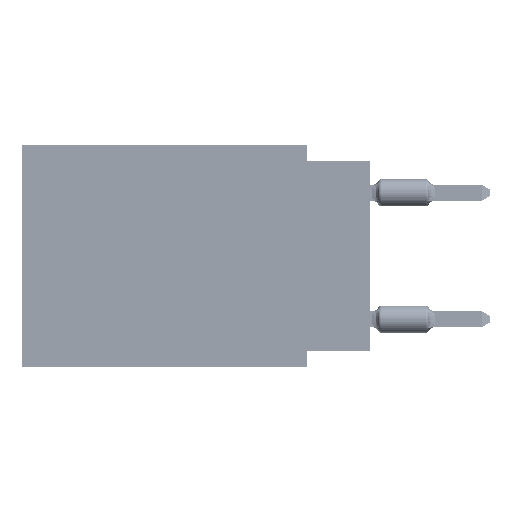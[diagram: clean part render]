
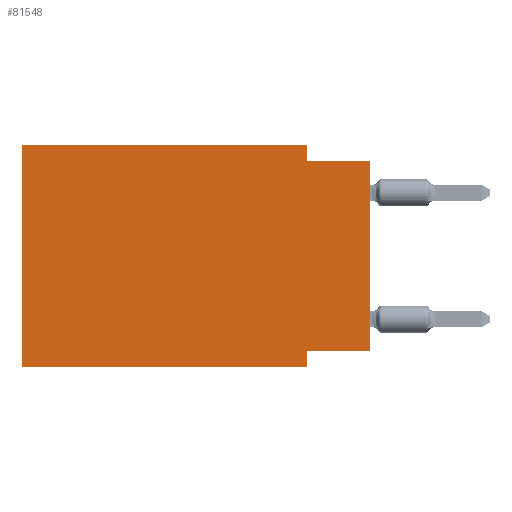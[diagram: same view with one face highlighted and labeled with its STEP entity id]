
A CAD part, left-side view. The second image highlights one B-rep face of the part: STEP entity #81548.
In plain terms, the highlighted planar face has unit normal (-1, 0, 0).
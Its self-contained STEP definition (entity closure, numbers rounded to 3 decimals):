
#2024 = ORIENTED_EDGE ( 'NONE', *, *, #3509, .F. ) ;
#3143 = AXIS2_PLACEMENT_3D ( 'NONE', #29264, #36992, #66428 ) ;
#3509 = EDGE_CURVE ( 'NONE', #34362, #30360, #39210, .T. ) ;
#3958 = EDGE_CURVE ( 'NONE', #67403, #28481, #68541, .T. ) ;
#7052 = FACE_OUTER_BOUND ( 'NONE', #92737, .T. ) ;
#7469 = CARTESIAN_POINT ( 'NONE',  ( 0., 2.54, 0. ) ) ;
#8849 = VERTEX_POINT ( 'NONE', #11582 ) ;
#9757 = LINE ( 'NONE', #38260, #19211 ) ;
#11582 = CARTESIAN_POINT ( 'NONE',  ( 0., 2.54, -8.255 ) ) ;
#16676 = DIRECTION ( 'NONE',  ( 0., -1., 0. ) ) ;
#19211 = VECTOR ( 'NONE', #69609, 1000. ) ;
#26315 = CARTESIAN_POINT ( 'NONE',  ( 0., 13.97, -8.89 ) ) ;
#27398 = EDGE_CURVE ( 'NONE', #8849, #62726, #47108, .T. ) ;
#28058 = ORIENTED_EDGE ( 'NONE', *, *, #45153, .T. ) ;
#28481 = VERTEX_POINT ( 'NONE', #76829 ) ;
#29264 = CARTESIAN_POINT ( 'NONE',  ( 0., 13.97, 0. ) ) ;
#30360 = VERTEX_POINT ( 'NONE', #59349 ) ;
#31973 = CARTESIAN_POINT ( 'NONE',  ( 0., 13.97, 0. ) ) ;
#32003 = CARTESIAN_POINT ( 'NONE',  ( 0., 2.54, 0. ) ) ;
#33080 = VERTEX_POINT ( 'NONE', #58321 ) ;
#34362 = VERTEX_POINT ( 'NONE', #39349 ) ;
#35108 = ORIENTED_EDGE ( 'NONE', *, *, #39375, .F. ) ;
#35407 = VECTOR ( 'NONE', #42680, 1000. ) ;
#36440 = VECTOR ( 'NONE', #90115, 1000. ) ;
#36992 = DIRECTION ( 'NONE',  ( 1., 0., 0. ) ) ;
#38260 = CARTESIAN_POINT ( 'NONE',  ( 0., 13.97, 0. ) ) ;
#38463 = CARTESIAN_POINT ( 'NONE',  ( 0., 2.54, -8.89 ) ) ;
#39210 = LINE ( 'NONE', #31973, #61762 ) ;
#39349 = CARTESIAN_POINT ( 'NONE',  ( 0., 13.97, -8.89 ) ) ;
#39375 = EDGE_CURVE ( 'NONE', #30360, #82063, #9757, .T. ) ;
#40189 = ORIENTED_EDGE ( 'NONE', *, *, #27398, .F. ) ;
#42680 = DIRECTION ( 'NONE',  ( 0., 1., 0. ) ) ;
#43485 = ORIENTED_EDGE ( 'NONE', *, *, #44630, .T. ) ;
#44630 = EDGE_CURVE ( 'NONE', #34362, #62726, #63002, .T. ) ;
#45153 = EDGE_CURVE ( 'NONE', #33080, #28481, #72029, .T. ) ;
#46510 = LINE ( 'NONE', #7469, #48890 ) ;
#47108 = LINE ( 'NONE', #38463, #36440 ) ;
#48890 = VECTOR ( 'NONE', #70161, 1000. ) ;
#56105 = ORIENTED_EDGE ( 'NONE', *, *, #71677, .F. ) ;
#56377 = VECTOR ( 'NONE', #85104, 1000. ) ;
#57176 = CARTESIAN_POINT ( 'NONE',  ( 0., 0., -8.255 ) ) ;
#58133 = CARTESIAN_POINT ( 'NONE',  ( 0., 2.54, -0.635 ) ) ;
#58214 = PLANE ( 'NONE',  #3143 ) ;
#58321 = CARTESIAN_POINT ( 'NONE',  ( 0., 0., -8.255 ) ) ;
#59349 = CARTESIAN_POINT ( 'NONE',  ( 0., 13.97, 0. ) ) ;
#59772 = ORIENTED_EDGE ( 'NONE', *, *, #76416, .F. ) ;
#61291 = CARTESIAN_POINT ( 'NONE',  ( 0., 0., -0.635 ) ) ;
#61762 = VECTOR ( 'NONE', #68650, 1000. ) ;
#62726 = VERTEX_POINT ( 'NONE', #63433 ) ;
#63002 = LINE ( 'NONE', #26315, #79534 ) ;
#63433 = CARTESIAN_POINT ( 'NONE',  ( 0., 2.54, -8.89 ) ) ;
#66320 = LINE ( 'NONE', #57176, #35407 ) ;
#66428 = DIRECTION ( 'NONE',  ( 0., 0., -1. ) ) ;
#67403 = VERTEX_POINT ( 'NONE', #58133 ) ;
#68541 = LINE ( 'NONE', #61291, #74178 ) ;
#68650 = DIRECTION ( 'NONE',  ( 0., 0., 1. ) ) ;
#69609 = DIRECTION ( 'NONE',  ( 0., -1., 0. ) ) ;
#70161 = DIRECTION ( 'NONE',  ( 0., 0., -1. ) ) ;
#71677 = EDGE_CURVE ( 'NONE', #33080, #8849, #66320, .T. ) ;
#72029 = LINE ( 'NONE', #94241, #56377 ) ;
#74178 = VECTOR ( 'NONE', #90757, 1000. ) ;
#76018 = ORIENTED_EDGE ( 'NONE', *, *, #3958, .F. ) ;
#76416 = EDGE_CURVE ( 'NONE', #82063, #67403, #46510, .T. ) ;
#76829 = CARTESIAN_POINT ( 'NONE',  ( 0., 0., -0.635 ) ) ;
#79534 = VECTOR ( 'NONE', #16676, 1000. ) ;
#81548 = ADVANCED_FACE ( 'NONE', ( #7052 ), #58214, .F. ) ;
#82063 = VERTEX_POINT ( 'NONE', #32003 ) ;
#85104 = DIRECTION ( 'NONE',  ( 0., 0., 1. ) ) ;
#90115 = DIRECTION ( 'NONE',  ( 0., 0., -1. ) ) ;
#90757 = DIRECTION ( 'NONE',  ( 0., -1., 0. ) ) ;
#92737 = EDGE_LOOP ( 'NONE', ( #28058, #76018, #59772, #35108, #2024, #43485, #40189, #56105 ) ) ;
#94241 = CARTESIAN_POINT ( 'NONE',  ( 0., 0., 0. ) ) ;
